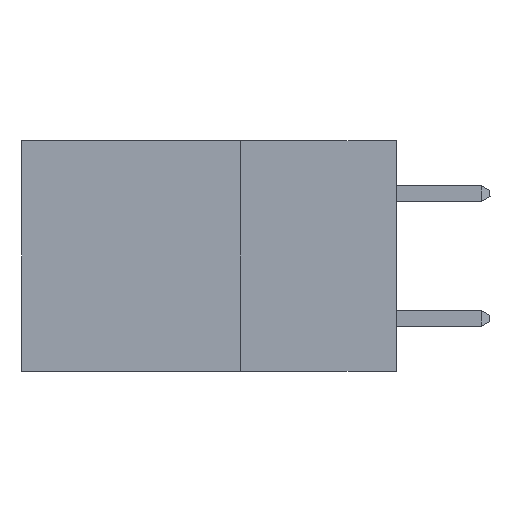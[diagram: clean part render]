
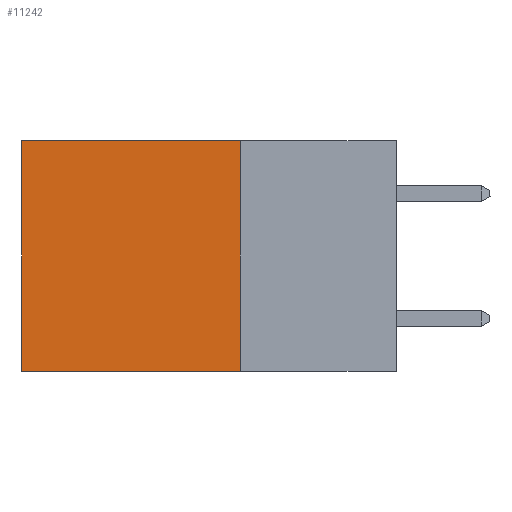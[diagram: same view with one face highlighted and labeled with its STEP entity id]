
A CAD part, left-side view. The second image highlights one B-rep face of the part: STEP entity #11242.
In plain terms, the highlighted planar face has unit normal (-1, 0, 0).
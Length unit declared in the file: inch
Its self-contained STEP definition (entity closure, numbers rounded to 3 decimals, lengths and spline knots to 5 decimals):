
#92 = CARTESIAN_POINT ( 'NONE',  ( 0.298, 0.25, 0. ) ) ;
#433 = ORIENTED_EDGE ( 'NONE', *, *, #8082, .T. ) ;
#834 = CARTESIAN_POINT ( 'NONE',  ( 0.298, 0.25, 0. ) ) ;
#2822 = EDGE_LOOP ( 'NONE', ( #6691, #13343, #5245, #433 ) ) ;
#2825 = CARTESIAN_POINT ( 'NONE',  ( 0.298, 0.6, -0.37 ) ) ;
#4549 = VECTOR ( 'NONE', #7392, 39.37008 ) ;
#4929 = VECTOR ( 'NONE', #8092, 39.37008 ) ;
#5245 = ORIENTED_EDGE ( 'NONE', *, *, #5681, .F. ) ;
#5681 = EDGE_CURVE ( 'NONE', #10667, #8334, #12765, .T. ) ;
#5765 = EDGE_CURVE ( 'NONE', #15030, #8407, #11618, .T. ) ;
#6008 = DIRECTION ( 'NONE',  ( 0., 0., -1. ) ) ;
#6669 = CARTESIAN_POINT ( 'NONE',  ( 0.298, 0.6, 0. ) ) ;
#6691 = ORIENTED_EDGE ( 'NONE', *, *, #5765, .T. ) ;
#7392 = DIRECTION ( 'NONE',  ( 0., 0., -1. ) ) ;
#8082 = EDGE_CURVE ( 'NONE', #10667, #15030, #10766, .T. ) ;
#8092 = DIRECTION ( 'NONE',  ( 0., 0., -1. ) ) ;
#8300 = DIRECTION ( 'NONE',  ( 0., 1., 0. ) ) ;
#8334 = VERTEX_POINT ( 'NONE', #9825 ) ;
#8407 = VERTEX_POINT ( 'NONE', #2825 ) ;
#8410 = CARTESIAN_POINT ( 'NONE',  ( 0.298, 0.25, 0. ) ) ;
#8438 = DIRECTION ( 'NONE',  ( 1., 0., 0. ) ) ;
#9151 = DIRECTION ( 'NONE',  ( 0., 1., 0. ) ) ;
#9825 = CARTESIAN_POINT ( 'NONE',  ( 0.298, 0.25, -0.37 ) ) ;
#10081 = CARTESIAN_POINT ( 'NONE',  ( 0.298, 0.25, 0. ) ) ;
#10435 = VECTOR ( 'NONE', #9151, 39.37008 ) ;
#10667 = VERTEX_POINT ( 'NONE', #10081 ) ;
#10766 = LINE ( 'NONE', #8410, #14773 ) ;
#11242 = ADVANCED_FACE ( 'NONE', ( #14857 ), #15680, .F. ) ;
#11618 = LINE ( 'NONE', #12355, #4549 ) ;
#12172 = LINE ( 'NONE', #14143, #10435 ) ;
#12355 = CARTESIAN_POINT ( 'NONE',  ( 0.298, 0.6, 0. ) ) ;
#12363 = EDGE_CURVE ( 'NONE', #8334, #8407, #12172, .T. ) ;
#12765 = LINE ( 'NONE', #834, #4929 ) ;
#13343 = ORIENTED_EDGE ( 'NONE', *, *, #12363, .F. ) ;
#14143 = CARTESIAN_POINT ( 'NONE',  ( 0.298, 0.25, -0.37 ) ) ;
#14264 = AXIS2_PLACEMENT_3D ( 'NONE', #92, #8438, #6008 ) ;
#14773 = VECTOR ( 'NONE', #8300, 39.37008 ) ;
#14857 = FACE_OUTER_BOUND ( 'NONE', #2822, .T. ) ;
#15030 = VERTEX_POINT ( 'NONE', #6669 ) ;
#15680 = PLANE ( 'NONE',  #14264 ) ;
